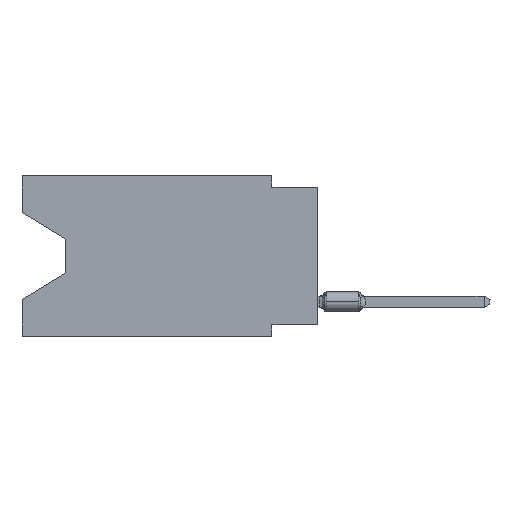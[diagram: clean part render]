
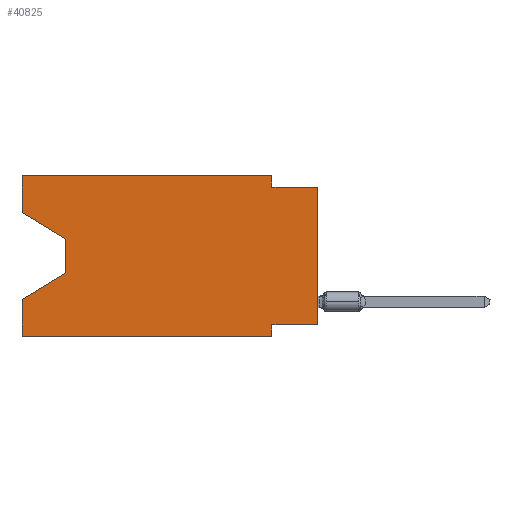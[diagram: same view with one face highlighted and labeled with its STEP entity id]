
A CAD part, left-side view. The second image highlights one B-rep face of the part: STEP entity #40825.
In plain terms, the highlighted planar face has unit normal (-1, 0, 0).
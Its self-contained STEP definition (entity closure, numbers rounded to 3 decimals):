
#160 = ORIENTED_EDGE ( 'NONE', *, *, #32558, .F. ) ;
#181 = VECTOR ( 'NONE', #4891, 1000. ) ;
#184 = DIRECTION ( 'NONE',  ( 0., 0., -1. ) ) ;
#333 = ORIENTED_EDGE ( 'NONE', *, *, #42511, .T. ) ;
#608 = FACE_OUTER_BOUND ( 'NONE', #32046, .T. ) ;
#1554 = VERTEX_POINT ( 'NONE', #24821 ) ;
#1923 = VERTEX_POINT ( 'NONE', #14645 ) ;
#2535 = CARTESIAN_POINT ( 'NONE',  ( 0., 0., 0. ) ) ;
#2896 = DIRECTION ( 'NONE',  ( 0., -1., 0. ) ) ;
#2964 = EDGE_CURVE ( 'NONE', #22114, #29345, #4372, .T. ) ;
#3127 = ORIENTED_EDGE ( 'NONE', *, *, #28645, .F. ) ;
#4007 = EDGE_CURVE ( 'NONE', #29016, #29345, #14434, .T. ) ;
#4372 = LINE ( 'NONE', #24236, #9659 ) ;
#4749 = CARTESIAN_POINT ( 'NONE',  ( 0., 16.383, -2.038 ) ) ;
#4891 = DIRECTION ( 'NONE',  ( 0., 0., -1. ) ) ;
#5093 = CARTESIAN_POINT ( 'NONE',  ( 0., 16.383, -8.89 ) ) ;
#5128 = DIRECTION ( 'NONE',  ( 0., 0., 1. ) ) ;
#5167 = CARTESIAN_POINT ( 'NONE',  ( 0., 13.97, -3.505 ) ) ;
#5207 = CARTESIAN_POINT ( 'NONE',  ( 0., 2.54, -8.89 ) ) ;
#5696 = DIRECTION ( 'NONE',  ( 0., -1., 0. ) ) ;
#5778 = ORIENTED_EDGE ( 'NONE', *, *, #12200, .F. ) ;
#6297 = LINE ( 'NONE', #2535, #9512 ) ;
#6425 = VERTEX_POINT ( 'NONE', #38034 ) ;
#6633 = EDGE_CURVE ( 'NONE', #26667, #16672, #15715, .T. ) ;
#7317 = ORIENTED_EDGE ( 'NONE', *, *, #2964, .T. ) ;
#7770 = DIRECTION ( 'NONE',  ( 0., -0.855, -0.519 ) ) ;
#8043 = DIRECTION ( 'NONE',  ( 0., -1., 0. ) ) ;
#9392 = VERTEX_POINT ( 'NONE', #41911 ) ;
#9512 = VECTOR ( 'NONE', #22390, 1000. ) ;
#9659 = VECTOR ( 'NONE', #31075, 1000. ) ;
#9950 = DIRECTION ( 'NONE',  ( 0., 1., 0. ) ) ;
#10733 = LINE ( 'NONE', #24183, #27925 ) ;
#11529 = CARTESIAN_POINT ( 'NONE',  ( 0., 16.383, -2.038 ) ) ;
#11587 = CARTESIAN_POINT ( 'NONE',  ( 0., 16.383, -8.89 ) ) ;
#12200 = EDGE_CURVE ( 'NONE', #1554, #1923, #29461, .T. ) ;
#12700 = DIRECTION ( 'NONE',  ( 0., 0., -1. ) ) ;
#14084 = PLANE ( 'NONE',  #42896 ) ;
#14434 = LINE ( 'NONE', #35362, #41333 ) ;
#14645 = CARTESIAN_POINT ( 'NONE',  ( 0., 2.54, -8.89 ) ) ;
#15715 = LINE ( 'NONE', #27148, #33029 ) ;
#16672 = VERTEX_POINT ( 'NONE', #43522 ) ;
#16798 = EDGE_CURVE ( 'NONE', #27263, #22114, #17718, .T. ) ;
#16890 = VECTOR ( 'NONE', #30797, 1000. ) ;
#17014 = LINE ( 'NONE', #30457, #23140 ) ;
#17137 = DIRECTION ( 'NONE',  ( 0., 0., -1. ) ) ;
#17718 = LINE ( 'NONE', #27635, #181 ) ;
#18005 = EDGE_CURVE ( 'NONE', #9392, #16672, #6297, .T. ) ;
#18700 = ORIENTED_EDGE ( 'NONE', *, *, #4007, .F. ) ;
#19999 = VERTEX_POINT ( 'NONE', #40007 ) ;
#20243 = CARTESIAN_POINT ( 'NONE',  ( 0., 16.383, 0. ) ) ;
#20473 = DIRECTION ( 'NONE',  ( 1., 0., 0. ) ) ;
#21230 = LINE ( 'NONE', #11529, #35158 ) ;
#22114 = VERTEX_POINT ( 'NONE', #31011 ) ;
#22390 = DIRECTION ( 'NONE',  ( 0., 0., 1. ) ) ;
#22448 = LINE ( 'NONE', #32829, #38882 ) ;
#23140 = VECTOR ( 'NONE', #9950, 1000. ) ;
#23348 = CARTESIAN_POINT ( 'NONE',  ( 0., 2.54, -0.635 ) ) ;
#24183 = CARTESIAN_POINT ( 'NONE',  ( 0., 2.54, 0. ) ) ;
#24236 = CARTESIAN_POINT ( 'NONE',  ( 0., 13.97, -5.385 ) ) ;
#24552 = VECTOR ( 'NONE', #8043, 1000. ) ;
#24729 = EDGE_CURVE ( 'NONE', #28661, #27263, #21230, .T. ) ;
#24821 = CARTESIAN_POINT ( 'NONE',  ( 0., 2.54, -8.255 ) ) ;
#26252 = ORIENTED_EDGE ( 'NONE', *, *, #18005, .T. ) ;
#26667 = VERTEX_POINT ( 'NONE', #23348 ) ;
#27148 = CARTESIAN_POINT ( 'NONE',  ( 0., 0., -0.635 ) ) ;
#27263 = VERTEX_POINT ( 'NONE', #5167 ) ;
#27635 = CARTESIAN_POINT ( 'NONE',  ( 0., 13.97, -3.505 ) ) ;
#27925 = VECTOR ( 'NONE', #17137, 1000. ) ;
#28173 = ORIENTED_EDGE ( 'NONE', *, *, #6633, .F. ) ;
#28645 = EDGE_CURVE ( 'NONE', #28661, #6425, #34990, .T. ) ;
#28661 = VERTEX_POINT ( 'NONE', #4749 ) ;
#29016 = VERTEX_POINT ( 'NONE', #5093 ) ;
#29223 = ORIENTED_EDGE ( 'NONE', *, *, #38142, .F. ) ;
#29345 = VERTEX_POINT ( 'NONE', #33972 ) ;
#29461 = LINE ( 'NONE', #5207, #33074 ) ;
#30139 = ORIENTED_EDGE ( 'NONE', *, *, #24729, .T. ) ;
#30457 = CARTESIAN_POINT ( 'NONE',  ( 0., 0., -8.255 ) ) ;
#30797 = DIRECTION ( 'NONE',  ( 0., 0., 1. ) ) ;
#31011 = CARTESIAN_POINT ( 'NONE',  ( 0., 13.97, -5.385 ) ) ;
#31075 = DIRECTION ( 'NONE',  ( 0., 0.855, -0.519 ) ) ;
#31248 = CARTESIAN_POINT ( 'NONE',  ( 0., 16.383, 0. ) ) ;
#31820 = ORIENTED_EDGE ( 'NONE', *, *, #40389, .F. ) ;
#32046 = EDGE_LOOP ( 'NONE', ( #30139, #38957, #7317, #18700, #333, #5778, #31820, #26252, #28173, #29223, #160, #3127 ) ) ;
#32558 = EDGE_CURVE ( 'NONE', #6425, #19999, #22448, .T. ) ;
#32829 = CARTESIAN_POINT ( 'NONE',  ( 0., 16.383, 0. ) ) ;
#33029 = VECTOR ( 'NONE', #2896, 1000. ) ;
#33074 = VECTOR ( 'NONE', #12700, 1000. ) ;
#33972 = CARTESIAN_POINT ( 'NONE',  ( 0., 16.383, -6.852 ) ) ;
#34312 = LINE ( 'NONE', #11587, #24552 ) ;
#34990 = LINE ( 'NONE', #31248, #16890 ) ;
#35158 = VECTOR ( 'NONE', #7770, 1000. ) ;
#35362 = CARTESIAN_POINT ( 'NONE',  ( 0., 16.383, 0. ) ) ;
#38034 = CARTESIAN_POINT ( 'NONE',  ( 0., 16.383, 0. ) ) ;
#38142 = EDGE_CURVE ( 'NONE', #19999, #26667, #10733, .T. ) ;
#38882 = VECTOR ( 'NONE', #5696, 1000. ) ;
#38957 = ORIENTED_EDGE ( 'NONE', *, *, #16798, .T. ) ;
#40007 = CARTESIAN_POINT ( 'NONE',  ( 0., 2.54, 0. ) ) ;
#40389 = EDGE_CURVE ( 'NONE', #9392, #1554, #17014, .T. ) ;
#40825 = ADVANCED_FACE ( 'NONE', ( #608 ), #14084, .F. ) ;
#41333 = VECTOR ( 'NONE', #5128, 1000. ) ;
#41911 = CARTESIAN_POINT ( 'NONE',  ( 0., 0., -8.255 ) ) ;
#42511 = EDGE_CURVE ( 'NONE', #29016, #1923, #34312, .T. ) ;
#42896 = AXIS2_PLACEMENT_3D ( 'NONE', #20243, #20473, #184 ) ;
#43522 = CARTESIAN_POINT ( 'NONE',  ( 0., 0., -0.635 ) ) ;
